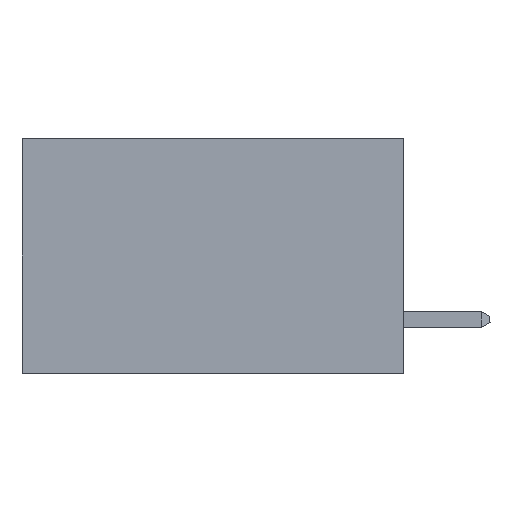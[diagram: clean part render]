
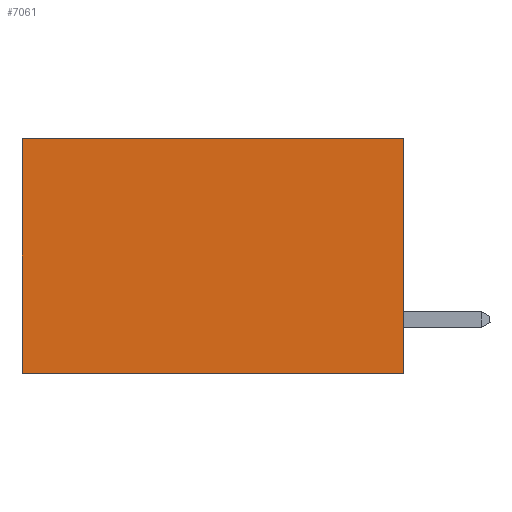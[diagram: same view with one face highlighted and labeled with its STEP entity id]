
A CAD part, left-side view. The second image highlights one B-rep face of the part: STEP entity #7061.
In plain terms, the highlighted planar face has unit normal (-1, 0, 0).
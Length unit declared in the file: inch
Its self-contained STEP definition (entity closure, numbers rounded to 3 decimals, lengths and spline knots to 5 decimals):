
#178 = VERTEX_POINT ( 'NONE', #11306 ) ;
#796 = DIRECTION ( 'NONE',  ( 0., 1., 0. ) ) ;
#1053 = EDGE_CURVE ( 'NONE', #19281, #178, #15005, .T. ) ;
#1558 = DIRECTION ( 'NONE',  ( 0., 0., -1. ) ) ;
#1991 = CARTESIAN_POINT ( 'NONE',  ( 0.2875, 0., -0.37 ) ) ;
#2146 = VERTEX_POINT ( 'NONE', #7376 ) ;
#2299 = VECTOR ( 'NONE', #796, 39.37008 ) ;
#2900 = VECTOR ( 'NONE', #1558, 39.37008 ) ;
#3205 = LINE ( 'NONE', #9562, #6987 ) ;
#4834 = CARTESIAN_POINT ( 'NONE',  ( 0.2875, 0., -0.37 ) ) ;
#5696 = CARTESIAN_POINT ( 'NONE',  ( 0.2875, 0., 0. ) ) ;
#5779 = ORIENTED_EDGE ( 'NONE', *, *, #1053, .F. ) ;
#6987 = VECTOR ( 'NONE', #17195, 39.37008 ) ;
#7061 = ADVANCED_FACE ( 'NONE', ( #18078 ), #16593, .F. ) ;
#7320 = DIRECTION ( 'NONE',  ( 1., 0., 0. ) ) ;
#7376 = CARTESIAN_POINT ( 'NONE',  ( 0.2875, 0.6, 0. ) ) ;
#7445 = CARTESIAN_POINT ( 'NONE',  ( 0.2875, 0., 0. ) ) ;
#7695 = LINE ( 'NONE', #14345, #2900 ) ;
#7904 = LINE ( 'NONE', #15578, #11591 ) ;
#7988 = EDGE_CURVE ( 'NONE', #13714, #19281, #3205, .T. ) ;
#8144 = EDGE_LOOP ( 'NONE', ( #15517, #5779, #17228, #10710 ) ) ;
#9412 = AXIS2_PLACEMENT_3D ( 'NONE', #5696, #7320, #18025 ) ;
#9562 = CARTESIAN_POINT ( 'NONE',  ( 0.2875, 0., 0. ) ) ;
#10710 = ORIENTED_EDGE ( 'NONE', *, *, #20150, .T. ) ;
#11306 = CARTESIAN_POINT ( 'NONE',  ( 0.2875, 0.6, -0.37 ) ) ;
#11591 = VECTOR ( 'NONE', #18432, 39.37008 ) ;
#13714 = VERTEX_POINT ( 'NONE', #7445 ) ;
#14345 = CARTESIAN_POINT ( 'NONE',  ( 0.2875, 0.6, 0. ) ) ;
#15005 = LINE ( 'NONE', #1991, #2299 ) ;
#15414 = EDGE_CURVE ( 'NONE', #2146, #178, #7695, .T. ) ;
#15517 = ORIENTED_EDGE ( 'NONE', *, *, #15414, .T. ) ;
#15578 = CARTESIAN_POINT ( 'NONE',  ( 0.2875, 0., 0. ) ) ;
#16593 = PLANE ( 'NONE',  #9412 ) ;
#17195 = DIRECTION ( 'NONE',  ( 0., 0., -1. ) ) ;
#17228 = ORIENTED_EDGE ( 'NONE', *, *, #7988, .F. ) ;
#18025 = DIRECTION ( 'NONE',  ( 0., 0., -1. ) ) ;
#18078 = FACE_OUTER_BOUND ( 'NONE', #8144, .T. ) ;
#18432 = DIRECTION ( 'NONE',  ( 0., 1., 0. ) ) ;
#19281 = VERTEX_POINT ( 'NONE', #4834 ) ;
#20150 = EDGE_CURVE ( 'NONE', #13714, #2146, #7904, .T. ) ;
